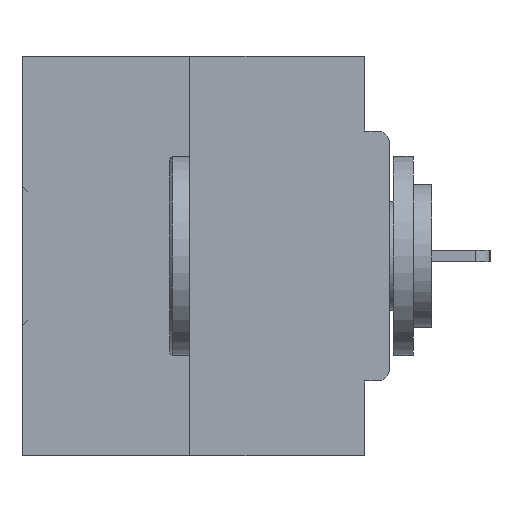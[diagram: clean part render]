
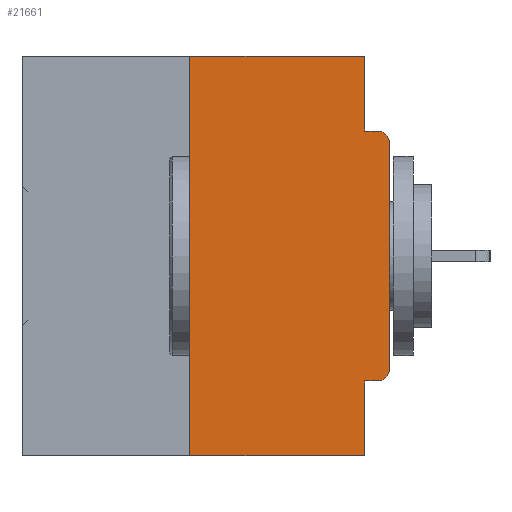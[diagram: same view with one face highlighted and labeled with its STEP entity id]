
A CAD part, left-side view. The second image highlights one B-rep face of the part: STEP entity #21661.
In plain terms, the highlighted planar face has unit normal (-1, 0, 0).
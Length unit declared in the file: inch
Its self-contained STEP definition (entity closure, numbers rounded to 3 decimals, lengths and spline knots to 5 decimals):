
#1274 = CARTESIAN_POINT ( 'NONE',  ( 0., 0.031, -0.4065 ) ) ;
#1438 = VECTOR ( 'NONE', #8008, 39.37008 ) ;
#1483 = AXIS2_PLACEMENT_3D ( 'NONE', #1764, #33475, #24175 ) ;
#1764 = CARTESIAN_POINT ( 'NONE',  ( 0., 0.015, -0.1085 ) ) ;
#2026 = EDGE_CURVE ( 'NONE', #33020, #40224, #25476, .T. ) ;
#2087 = CARTESIAN_POINT ( 'NONE',  ( 0., 0., -0.3915 ) ) ;
#2167 = EDGE_CURVE ( 'NONE', #35952, #35681, #22992, .T. ) ;
#2706 = ORIENTED_EDGE ( 'NONE', *, *, #2026, .F. ) ;
#2903 = VERTEX_POINT ( 'NONE', #15526 ) ;
#2942 = LINE ( 'NONE', #24047, #13854 ) ;
#3198 = ORIENTED_EDGE ( 'NONE', *, *, #18345, .F. ) ;
#3590 = CARTESIAN_POINT ( 'NONE',  ( 0., 0.031, -0.0935 ) ) ;
#4300 = VERTEX_POINT ( 'NONE', #2087 ) ;
#4367 = DIRECTION ( 'NONE',  ( 0., 0., -1. ) ) ;
#5218 = EDGE_CURVE ( 'NONE', #15573, #35681, #37108, .T. ) ;
#5761 = ORIENTED_EDGE ( 'NONE', *, *, #37709, .F. ) ;
#6036 = EDGE_CURVE ( 'NONE', #4300, #2903, #36035, .T. ) ;
#6529 = DIRECTION ( 'NONE',  ( 1., 0., 0. ) ) ;
#8008 = DIRECTION ( 'NONE',  ( 0., -1., 0. ) ) ;
#8145 = CARTESIAN_POINT ( 'NONE',  ( 0., 0.015, -0.3915 ) ) ;
#8867 = VECTOR ( 'NONE', #16622, 39.37008 ) ;
#9031 = FACE_OUTER_BOUND ( 'NONE', #38668, .T. ) ;
#9996 = PLANE ( 'NONE',  #33702 ) ;
#10379 = LINE ( 'NONE', #26790, #1438 ) ;
#10528 = ORIENTED_EDGE ( 'NONE', *, *, #37758, .F. ) ;
#10888 = CARTESIAN_POINT ( 'NONE',  ( 0., 0.015, -0.0935 ) ) ;
#11358 = DIRECTION ( 'NONE',  ( 0., 0., -1. ) ) ;
#11518 = DIRECTION ( 'NONE',  ( 0., 1., 0. ) ) ;
#11705 = DIRECTION ( 'NONE',  ( 0., -1., 0. ) ) ;
#11944 = VECTOR ( 'NONE', #11705, 39.37008 ) ;
#12168 = ORIENTED_EDGE ( 'NONE', *, *, #2167, .F. ) ;
#13053 = CARTESIAN_POINT ( 'NONE',  ( 0., 0.031, -0.5 ) ) ;
#13854 = VECTOR ( 'NONE', #11518, 39.37008 ) ;
#14715 = VERTEX_POINT ( 'NONE', #25552 ) ;
#15526 = CARTESIAN_POINT ( 'NONE',  ( 0., 0., -0.1085 ) ) ;
#15573 = VERTEX_POINT ( 'NONE', #20135 ) ;
#15805 = LINE ( 'NONE', #32895, #40038 ) ;
#16622 = DIRECTION ( 'NONE',  ( 0., 0., 1. ) ) ;
#16772 = CIRCLE ( 'NONE', #37110, 0.015 ) ;
#17038 = VECTOR ( 'NONE', #21912, 39.37008 ) ;
#17053 = DIRECTION ( 'NONE',  ( 0., 0., -1. ) ) ;
#17906 = ORIENTED_EDGE ( 'NONE', *, *, #32046, .T. ) ;
#18345 = EDGE_CURVE ( 'NONE', #28033, #14715, #10379, .T. ) ;
#19167 = CARTESIAN_POINT ( 'NONE',  ( 0., 0.46, -0.5 ) ) ;
#19223 = CARTESIAN_POINT ( 'NONE',  ( 0., 0.46, 0. ) ) ;
#20100 = CARTESIAN_POINT ( 'NONE',  ( 0., 0.031, -0.5 ) ) ;
#20135 = CARTESIAN_POINT ( 'NONE',  ( 0., 0.25, -0.5 ) ) ;
#20251 = DIRECTION ( 'NONE',  ( -1., 0., 0. ) ) ;
#20723 = LINE ( 'NONE', #30252, #35585 ) ;
#21450 = ORIENTED_EDGE ( 'NONE', *, *, #26497, .F. ) ;
#21661 = ADVANCED_FACE ( 'NONE', ( #9031 ), #9996, .F. ) ;
#21912 = DIRECTION ( 'NONE',  ( 0., -1., 0. ) ) ;
#22388 = DIRECTION ( 'NONE',  ( 0., 0., -1. ) ) ;
#22992 = LINE ( 'NONE', #20100, #31966 ) ;
#24047 = CARTESIAN_POINT ( 'NONE',  ( 0., 0., -0.4065 ) ) ;
#24175 = DIRECTION ( 'NONE',  ( 0., 0., -1. ) ) ;
#25476 = LINE ( 'NONE', #40867, #17038 ) ;
#25552 = CARTESIAN_POINT ( 'NONE',  ( 0., 0.031, 0. ) ) ;
#26497 = EDGE_CURVE ( 'NONE', #26778, #35952, #2942, .T. ) ;
#26556 = EDGE_CURVE ( 'NONE', #2903, #40224, #28184, .T. ) ;
#26663 = DIRECTION ( 'NONE',  ( 0., 0., 1. ) ) ;
#26778 = VERTEX_POINT ( 'NONE', #32308 ) ;
#26790 = CARTESIAN_POINT ( 'NONE',  ( 0., 0.46, 0. ) ) ;
#26872 = ORIENTED_EDGE ( 'NONE', *, *, #6036, .T. ) ;
#28033 = VERTEX_POINT ( 'NONE', #37464 ) ;
#28184 = CIRCLE ( 'NONE', #1483, 0.015 ) ;
#29372 = ORIENTED_EDGE ( 'NONE', *, *, #26556, .T. ) ;
#30252 = CARTESIAN_POINT ( 'NONE',  ( 0., 0.031, 0. ) ) ;
#30335 = ORIENTED_EDGE ( 'NONE', *, *, #5218, .T. ) ;
#31966 = VECTOR ( 'NONE', #17053, 39.37008 ) ;
#32046 = EDGE_CURVE ( 'NONE', #26778, #4300, #16772, .T. ) ;
#32308 = CARTESIAN_POINT ( 'NONE',  ( 0., 0.015, -0.4065 ) ) ;
#32895 = CARTESIAN_POINT ( 'NONE',  ( 0., 0.25, 0. ) ) ;
#33020 = VERTEX_POINT ( 'NONE', #3590 ) ;
#33475 = DIRECTION ( 'NONE',  ( -1., 0., 0. ) ) ;
#33702 = AXIS2_PLACEMENT_3D ( 'NONE', #19223, #6529, #22388 ) ;
#35585 = VECTOR ( 'NONE', #11358, 39.37008 ) ;
#35588 = CARTESIAN_POINT ( 'NONE',  ( 0., 0., 0. ) ) ;
#35681 = VERTEX_POINT ( 'NONE', #13053 ) ;
#35952 = VERTEX_POINT ( 'NONE', #1274 ) ;
#36035 = LINE ( 'NONE', #35588, #8867 ) ;
#37108 = LINE ( 'NONE', #19167, #11944 ) ;
#37110 = AXIS2_PLACEMENT_3D ( 'NONE', #8145, #20251, #4367 ) ;
#37464 = CARTESIAN_POINT ( 'NONE',  ( 0., 0.25, 0. ) ) ;
#37709 = EDGE_CURVE ( 'NONE', #15573, #28033, #15805, .T. ) ;
#37758 = EDGE_CURVE ( 'NONE', #14715, #33020, #20723, .T. ) ;
#38668 = EDGE_LOOP ( 'NONE', ( #3198, #5761, #30335, #12168, #21450, #17906, #26872, #29372, #2706, #10528 ) ) ;
#40038 = VECTOR ( 'NONE', #26663, 39.37008 ) ;
#40224 = VERTEX_POINT ( 'NONE', #10888 ) ;
#40867 = CARTESIAN_POINT ( 'NONE',  ( 0., 0., -0.0935 ) ) ;
